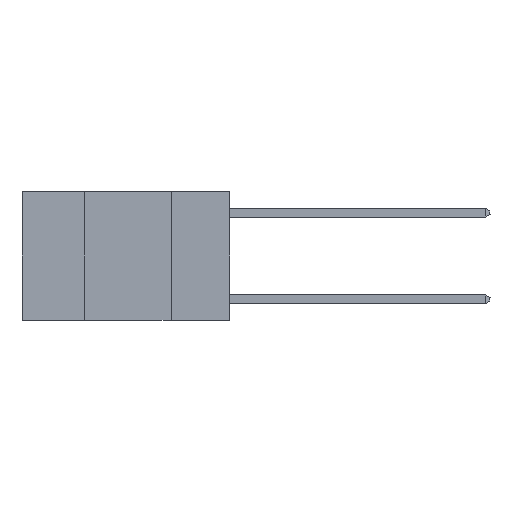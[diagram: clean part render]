
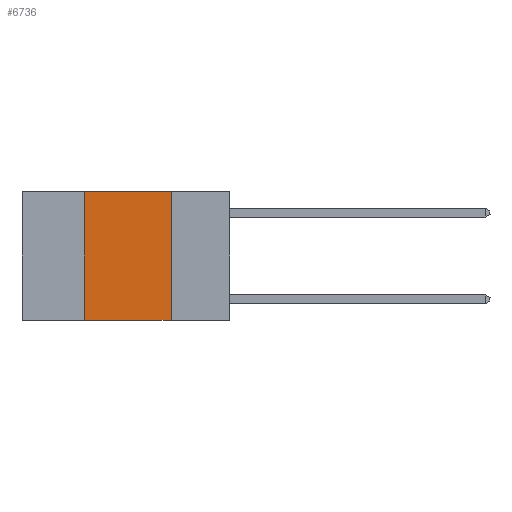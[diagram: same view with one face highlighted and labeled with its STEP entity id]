
A CAD part, left-side view. The second image highlights one B-rep face of the part: STEP entity #6736.
In plain terms, the highlighted planar face has unit normal (-1, 0, 0).
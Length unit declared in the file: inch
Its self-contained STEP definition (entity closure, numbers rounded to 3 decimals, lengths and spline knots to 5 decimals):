
#1359 = EDGE_CURVE ( 'NONE', #3998, #9450, #24676, .T. ) ;
#1483 = VECTOR ( 'NONE', #25694, 39.37008 ) ;
#2516 = VECTOR ( 'NONE', #6675, 39.37008 ) ;
#3608 = LINE ( 'NONE', #15739, #1483 ) ;
#3998 = VERTEX_POINT ( 'NONE', #10293 ) ;
#4208 = ORIENTED_EDGE ( 'NONE', *, *, #17665, .T. ) ;
#5188 = ORIENTED_EDGE ( 'NONE', *, *, #20416, .F. ) ;
#5688 = VECTOR ( 'NONE', #23530, 39.37008 ) ;
#6675 = DIRECTION ( 'NONE',  ( 0., 0., -1. ) ) ;
#6736 = ADVANCED_FACE ( 'NONE', ( #18051 ), #7995, .F. ) ;
#6953 = CARTESIAN_POINT ( 'NONE',  ( 0., 0.17, -0.37 ) ) ;
#7881 = DIRECTION ( 'NONE',  ( 1., 0., 0. ) ) ;
#7995 = PLANE ( 'NONE',  #14580 ) ;
#8095 = CARTESIAN_POINT ( 'NONE',  ( 0., 0.6, -0.37 ) ) ;
#9275 = ORIENTED_EDGE ( 'NONE', *, *, #13824, .F. ) ;
#9450 = VERTEX_POINT ( 'NONE', #6953 ) ;
#9825 = DIRECTION ( 'NONE',  ( 0., 0., -1. ) ) ;
#10293 = CARTESIAN_POINT ( 'NONE',  ( 0., 0.17, 0. ) ) ;
#10662 = CARTESIAN_POINT ( 'NONE',  ( 0., 0.42, -0.37 ) ) ;
#11346 = LINE ( 'NONE', #8095, #22590 ) ;
#13824 = EDGE_CURVE ( 'NONE', #24378, #3998, #25575, .T. ) ;
#13967 = EDGE_LOOP ( 'NONE', ( #18452, #9275, #5188, #4208 ) ) ;
#14505 = CARTESIAN_POINT ( 'NONE',  ( 0., 0.42, 0. ) ) ;
#14580 = AXIS2_PLACEMENT_3D ( 'NONE', #20386, #7881, #9825 ) ;
#15491 = CARTESIAN_POINT ( 'NONE',  ( 0., 0.6, 0. ) ) ;
#15739 = CARTESIAN_POINT ( 'NONE',  ( 0., 0.42, 0. ) ) ;
#17083 = CARTESIAN_POINT ( 'NONE',  ( 0., 0.17, 0. ) ) ;
#17665 = EDGE_CURVE ( 'NONE', #18062, #9450, #11346, .T. ) ;
#18051 = FACE_OUTER_BOUND ( 'NONE', #13967, .T. ) ;
#18062 = VERTEX_POINT ( 'NONE', #10662 ) ;
#18452 = ORIENTED_EDGE ( 'NONE', *, *, #1359, .F. ) ;
#20386 = CARTESIAN_POINT ( 'NONE',  ( 0., 0.6, 0. ) ) ;
#20416 = EDGE_CURVE ( 'NONE', #18062, #24378, #3608, .T. ) ;
#22590 = VECTOR ( 'NONE', #25723, 39.37008 ) ;
#23530 = DIRECTION ( 'NONE',  ( 0., -1., 0. ) ) ;
#24378 = VERTEX_POINT ( 'NONE', #14505 ) ;
#24676 = LINE ( 'NONE', #17083, #2516 ) ;
#25575 = LINE ( 'NONE', #15491, #5688 ) ;
#25694 = DIRECTION ( 'NONE',  ( 0., 0., 1. ) ) ;
#25723 = DIRECTION ( 'NONE',  ( 0., -1., 0. ) ) ;
